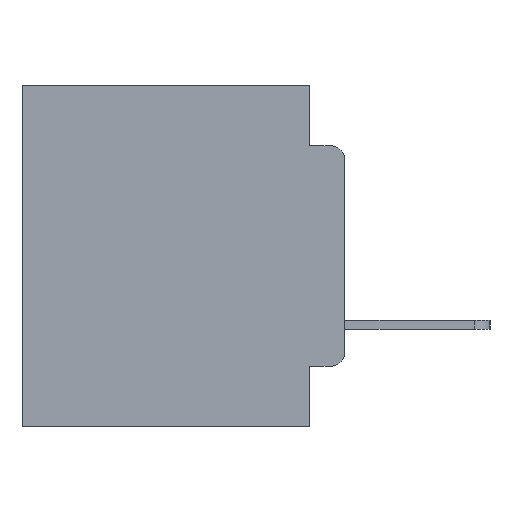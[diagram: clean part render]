
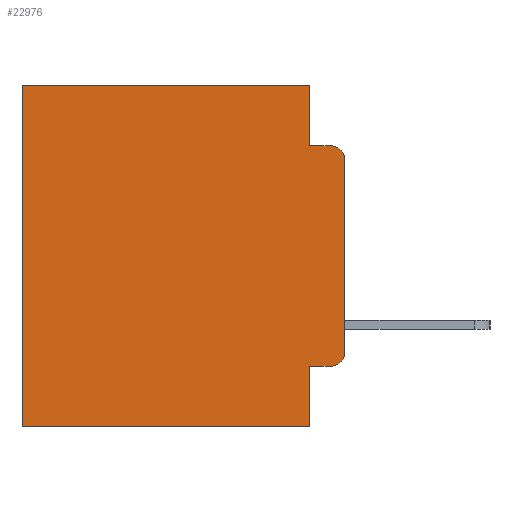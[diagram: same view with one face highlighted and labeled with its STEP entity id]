
A CAD part, left-side view. The second image highlights one B-rep face of the part: STEP entity #22976.
In plain terms, the highlighted planar face has unit normal (-1, 0, 0).
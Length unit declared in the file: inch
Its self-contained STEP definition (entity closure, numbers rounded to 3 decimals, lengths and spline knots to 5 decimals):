
#84 = DIRECTION ( 'NONE',  ( 0., 0., -1. ) ) ;
#266 = EDGE_CURVE ( 'NONE', #27165, #17491, #21314, .T. ) ;
#798 = VERTEX_POINT ( 'NONE', #23773 ) ;
#1100 = EDGE_LOOP ( 'NONE', ( #20193, #4884, #24852, #17486, #3534, #26878, #20330, #11977, #7206, #14101 ) ) ;
#1629 = DIRECTION ( 'NONE',  ( -1., 0., 0. ) ) ;
#1683 = VERTEX_POINT ( 'NONE', #14983 ) ;
#2141 = CARTESIAN_POINT ( 'NONE',  ( 0.298, 0., -0.1085 ) ) ;
#2329 = EDGE_CURVE ( 'NONE', #1683, #17979, #19987, .T. ) ;
#3204 = DIRECTION ( 'NONE',  ( 0., -1., 0. ) ) ;
#3534 = ORIENTED_EDGE ( 'NONE', *, *, #11016, .T. ) ;
#3846 = FACE_OUTER_BOUND ( 'NONE', #1100, .T. ) ;
#4545 = VECTOR ( 'NONE', #26598, 39.37008 ) ;
#4657 = VECTOR ( 'NONE', #84, 39.37008 ) ;
#4717 = VECTOR ( 'NONE', #10476, 39.37008 ) ;
#4848 = VECTOR ( 'NONE', #19380, 39.37008 ) ;
#4875 = CARTESIAN_POINT ( 'NONE',  ( 0.298, 0., -0.3915 ) ) ;
#4884 = ORIENTED_EDGE ( 'NONE', *, *, #266, .T. ) ;
#5638 = DIRECTION ( 'NONE',  ( 0., -1., 0. ) ) ;
#5643 = EDGE_CURVE ( 'NONE', #13825, #8910, #17080, .T. ) ;
#6255 = EDGE_CURVE ( 'NONE', #9067, #8910, #20777, .T. ) ;
#6403 = VECTOR ( 'NONE', #8063, 39.37008 ) ;
#6699 = LINE ( 'NONE', #27658, #12900 ) ;
#7124 = CARTESIAN_POINT ( 'NONE',  ( 0.298, 0.473, -0.5 ) ) ;
#7206 = ORIENTED_EDGE ( 'NONE', *, *, #2329, .T. ) ;
#7535 = AXIS2_PLACEMENT_3D ( 'NONE', #14190, #9666, #25116 ) ;
#8063 = DIRECTION ( 'NONE',  ( 0., 0., -1. ) ) ;
#8259 = AXIS2_PLACEMENT_3D ( 'NONE', #15548, #1629, #17796 ) ;
#8910 = VERTEX_POINT ( 'NONE', #7124 ) ;
#9067 = VERTEX_POINT ( 'NONE', #21234 ) ;
#9666 = DIRECTION ( 'NONE',  ( 1., 0., 0. ) ) ;
#9718 = CARTESIAN_POINT ( 'NONE',  ( 0.298, 0.02, -0.1085 ) ) ;
#10476 = DIRECTION ( 'NONE',  ( 0., 1., 0. ) ) ;
#10946 = LINE ( 'NONE', #17211, #4717 ) ;
#11016 = EDGE_CURVE ( 'NONE', #798, #13825, #10946, .T. ) ;
#11041 = CARTESIAN_POINT ( 'NONE',  ( 0.298, 0.02, -0.4115 ) ) ;
#11205 = CARTESIAN_POINT ( 'NONE',  ( 0.298, 0.473, 0. ) ) ;
#11919 = EDGE_CURVE ( 'NONE', #798, #13398, #16185, .T. ) ;
#11977 = ORIENTED_EDGE ( 'NONE', *, *, #26826, .F. ) ;
#12539 = DIRECTION ( 'NONE',  ( 0., 1., 0. ) ) ;
#12592 = LINE ( 'NONE', #21544, #6403 ) ;
#12900 = VECTOR ( 'NONE', #5638, 39.37008 ) ;
#13248 = DIRECTION ( 'NONE',  ( -1., 0., 0. ) ) ;
#13398 = VERTEX_POINT ( 'NONE', #27075 ) ;
#13825 = VERTEX_POINT ( 'NONE', #11205 ) ;
#14101 = ORIENTED_EDGE ( 'NONE', *, *, #19225, .T. ) ;
#14115 = CARTESIAN_POINT ( 'NONE',  ( 0.298, 0.051, 0. ) ) ;
#14190 = CARTESIAN_POINT ( 'NONE',  ( 0.298, 0., 0. ) ) ;
#14925 = CARTESIAN_POINT ( 'NONE',  ( 0.298, 0.473, 0. ) ) ;
#14983 = CARTESIAN_POINT ( 'NONE',  ( 0.298, 0.051, -0.4115 ) ) ;
#15548 = CARTESIAN_POINT ( 'NONE',  ( 0.298, 0.02, -0.3915 ) ) ;
#16185 = LINE ( 'NONE', #14115, #4657 ) ;
#16429 = CIRCLE ( 'NONE', #8259, 0.02 ) ;
#17080 = LINE ( 'NONE', #14925, #4848 ) ;
#17211 = CARTESIAN_POINT ( 'NONE',  ( 0.298, 0., 0. ) ) ;
#17486 = ORIENTED_EDGE ( 'NONE', *, *, #11919, .F. ) ;
#17491 = VERTEX_POINT ( 'NONE', #24711 ) ;
#17570 = DIRECTION ( 'NONE',  ( 0., 0., -1. ) ) ;
#17796 = DIRECTION ( 'NONE',  ( 0., 0., -1. ) ) ;
#17979 = VERTEX_POINT ( 'NONE', #11041 ) ;
#19225 = EDGE_CURVE ( 'NONE', #17979, #22963, #16429, .T. ) ;
#19380 = DIRECTION ( 'NONE',  ( 0., 0., -1. ) ) ;
#19987 = LINE ( 'NONE', #27443, #24982 ) ;
#20193 = ORIENTED_EDGE ( 'NONE', *, *, #27102, .F. ) ;
#20330 = ORIENTED_EDGE ( 'NONE', *, *, #6255, .F. ) ;
#20777 = LINE ( 'NONE', #27634, #25111 ) ;
#20826 = PLANE ( 'NONE',  #7535 ) ;
#21234 = CARTESIAN_POINT ( 'NONE',  ( 0.298, 0.051, -0.5 ) ) ;
#21314 = CIRCLE ( 'NONE', #25955, 0.02 ) ;
#21544 = CARTESIAN_POINT ( 'NONE',  ( 0.298, 0.051, 0. ) ) ;
#22566 = LINE ( 'NONE', #24525, #4545 ) ;
#22963 = VERTEX_POINT ( 'NONE', #4875 ) ;
#22976 = ADVANCED_FACE ( 'NONE', ( #3846 ), #20826, .F. ) ;
#23706 = EDGE_CURVE ( 'NONE', #13398, #17491, #6699, .T. ) ;
#23773 = CARTESIAN_POINT ( 'NONE',  ( 0.298, 0.051, 0. ) ) ;
#24525 = CARTESIAN_POINT ( 'NONE',  ( 0.298, 0., 0. ) ) ;
#24711 = CARTESIAN_POINT ( 'NONE',  ( 0.298, 0.02, -0.0885 ) ) ;
#24852 = ORIENTED_EDGE ( 'NONE', *, *, #23706, .F. ) ;
#24982 = VECTOR ( 'NONE', #3204, 39.37008 ) ;
#25111 = VECTOR ( 'NONE', #12539, 39.37008 ) ;
#25116 = DIRECTION ( 'NONE',  ( 0., 0., -1. ) ) ;
#25955 = AXIS2_PLACEMENT_3D ( 'NONE', #9718, #13248, #17570 ) ;
#26598 = DIRECTION ( 'NONE',  ( 0., 0., -1. ) ) ;
#26826 = EDGE_CURVE ( 'NONE', #1683, #9067, #12592, .T. ) ;
#26878 = ORIENTED_EDGE ( 'NONE', *, *, #5643, .T. ) ;
#27075 = CARTESIAN_POINT ( 'NONE',  ( 0.298, 0.051, -0.0885 ) ) ;
#27102 = EDGE_CURVE ( 'NONE', #27165, #22963, #22566, .T. ) ;
#27165 = VERTEX_POINT ( 'NONE', #2141 ) ;
#27443 = CARTESIAN_POINT ( 'NONE',  ( 0.298, 0.051, -0.4115 ) ) ;
#27634 = CARTESIAN_POINT ( 'NONE',  ( 0.298, 0., -0.5 ) ) ;
#27658 = CARTESIAN_POINT ( 'NONE',  ( 0.298, 0.051, -0.0885 ) ) ;
